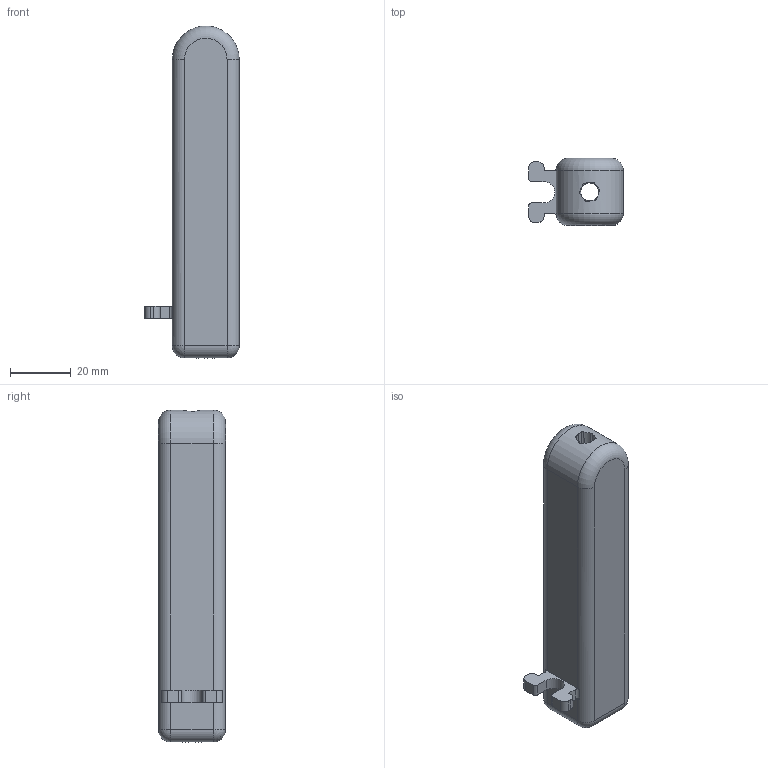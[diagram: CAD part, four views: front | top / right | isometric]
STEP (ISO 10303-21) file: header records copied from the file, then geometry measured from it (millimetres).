
FILE_DESCRIPTION((''),'2;1');
FILE_NAME('PM422Barrel2v3.stp','2015-08-22T19:08:37',('JamesRPatrick'),(''),'Autodesk Inventor 2012','Autodesk Inventor 2012','');
FILE_SCHEMA(('AUTOMOTIVE_DESIGN { 1 0 10303 214 1 1 1 1 }'));
Length unit declared in the file: millimetre
Products named in the file (1): PM422Barrel2v3
Bounding box: 31 x 22 x 109 mm (x, y, z)
Volume: 46795.4 mm3; surface area: 11844.6 mm2
Topology: 1 solids, 1 shells, 69 faces, 178 edges, 110 vertices
Faces by surface type: cylinder 24, plane 24, bspline 15, sphere 4, torus 2
Entity records: 2971 total; most frequent: CARTESIAN_POINT 1402, ORIENTED_EDGE 350, DIRECTION 280, EDGE_CURVE 175, AXIS2_PLACEMENT_3D 109, VERTEX_POINT 108, EDGE_LOOP 71, FACE_OUTER_BOUND 69
